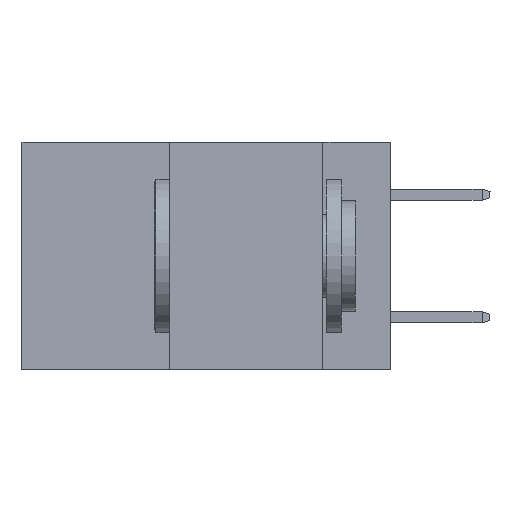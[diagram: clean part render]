
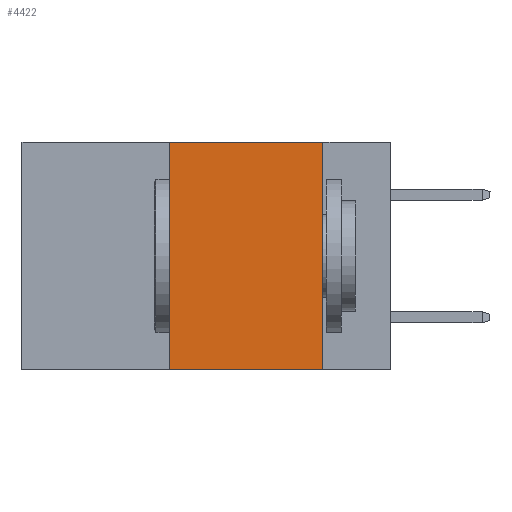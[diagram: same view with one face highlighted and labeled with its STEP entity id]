
A CAD part, left-side view. The second image highlights one B-rep face of the part: STEP entity #4422.
In plain terms, the highlighted planar face has unit normal (-1, 0, 0).
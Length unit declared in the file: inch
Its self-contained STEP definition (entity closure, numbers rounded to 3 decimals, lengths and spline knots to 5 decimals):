
#227 = EDGE_CURVE ( 'NONE', #2054, #19437, #1079, .T. ) ;
#306 = VECTOR ( 'NONE', #15755, 39.37008 ) ;
#491 = VECTOR ( 'NONE', #17191, 39.37008 ) ;
#1069 = DIRECTION ( 'NONE',  ( 0., 0., -1. ) ) ;
#1079 = LINE ( 'NONE', #17608, #491 ) ;
#1082 = ORIENTED_EDGE ( 'NONE', *, *, #15441, .T. ) ;
#1113 = ORIENTED_EDGE ( 'NONE', *, *, #1275, .F. ) ;
#1213 = EDGE_CURVE ( 'NONE', #18257, #2054, #17698, .T. ) ;
#1275 = EDGE_CURVE ( 'NONE', #19437, #13561, #7169, .T. ) ;
#1374 = CARTESIAN_POINT ( 'NONE',  ( 0., 0.11, 0. ) ) ;
#2054 = VERTEX_POINT ( 'NONE', #2754 ) ;
#2754 = CARTESIAN_POINT ( 'NONE',  ( 0., 0.36, 0. ) ) ;
#2980 = DIRECTION ( 'NONE',  ( 0., 0., 1. ) ) ;
#3446 = CARTESIAN_POINT ( 'NONE',  ( 0., 0.36, 0. ) ) ;
#4237 = AXIS2_PLACEMENT_3D ( 'NONE', #13632, #20822, #10148 ) ;
#4422 = ADVANCED_FACE ( 'NONE', ( #8786 ), #4614, .F. ) ;
#4614 = PLANE ( 'NONE',  #4237 ) ;
#5168 = LINE ( 'NONE', #8659, #306 ) ;
#6115 = CARTESIAN_POINT ( 'NONE',  ( 0., 0.11, 0. ) ) ;
#6569 = VECTOR ( 'NONE', #1069, 39.37008 ) ;
#6982 = ORIENTED_EDGE ( 'NONE', *, *, #1213, .F. ) ;
#7126 = ORIENTED_EDGE ( 'NONE', *, *, #227, .F. ) ;
#7169 = LINE ( 'NONE', #1374, #6569 ) ;
#8659 = CARTESIAN_POINT ( 'NONE',  ( 0., 0.6, -0.37 ) ) ;
#8786 = FACE_OUTER_BOUND ( 'NONE', #18187, .T. ) ;
#10148 = DIRECTION ( 'NONE',  ( 0., 0., -1. ) ) ;
#11544 = CARTESIAN_POINT ( 'NONE',  ( 0., 0.11, -0.37 ) ) ;
#12446 = VECTOR ( 'NONE', #2980, 39.37008 ) ;
#13561 = VERTEX_POINT ( 'NONE', #11544 ) ;
#13632 = CARTESIAN_POINT ( 'NONE',  ( 0., 0.6, 0. ) ) ;
#15441 = EDGE_CURVE ( 'NONE', #18257, #13561, #5168, .T. ) ;
#15755 = DIRECTION ( 'NONE',  ( 0., -1., 0. ) ) ;
#17191 = DIRECTION ( 'NONE',  ( 0., -1., 0. ) ) ;
#17608 = CARTESIAN_POINT ( 'NONE',  ( 0., 0.6, 0. ) ) ;
#17698 = LINE ( 'NONE', #3446, #12446 ) ;
#18187 = EDGE_LOOP ( 'NONE', ( #1113, #7126, #6982, #1082 ) ) ;
#18257 = VERTEX_POINT ( 'NONE', #20448 ) ;
#19437 = VERTEX_POINT ( 'NONE', #6115 ) ;
#20448 = CARTESIAN_POINT ( 'NONE',  ( 0., 0.36, -0.37 ) ) ;
#20822 = DIRECTION ( 'NONE',  ( 1., 0., 0. ) ) ;
